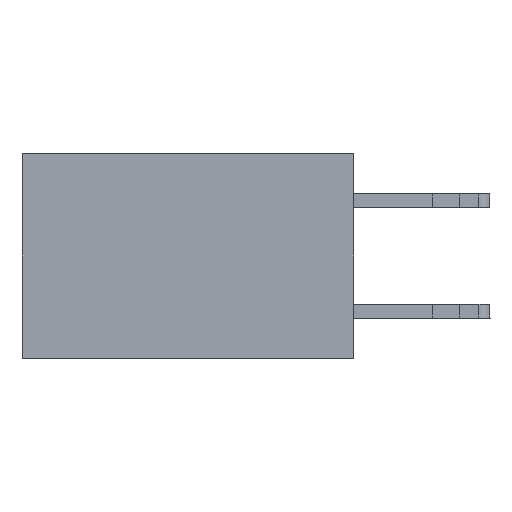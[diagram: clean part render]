
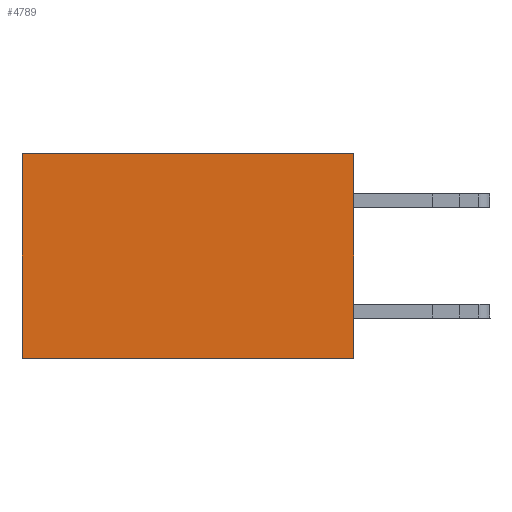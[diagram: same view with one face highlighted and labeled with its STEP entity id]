
A CAD part, left-side view. The second image highlights one B-rep face of the part: STEP entity #4789.
In plain terms, the highlighted planar face has unit normal (-1, 0, 0).
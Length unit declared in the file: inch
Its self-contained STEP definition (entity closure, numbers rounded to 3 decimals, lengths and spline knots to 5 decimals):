
#3145 = DIRECTION ( 'NONE',  ( 0., 1., 0. ) ) ;
#4263 = LINE ( 'NONE', #24356, #29850 ) ;
#4789 = ADVANCED_FACE ( 'NONE', ( #10942 ), #8909, .F. ) ;
#4837 = VERTEX_POINT ( 'NONE', #10345 ) ;
#5083 = LINE ( 'NONE', #15613, #27412 ) ;
#5341 = ORIENTED_EDGE ( 'NONE', *, *, #18465, .F. ) ;
#5527 = DIRECTION ( 'NONE',  ( 0., 0., -1. ) ) ;
#6210 = CARTESIAN_POINT ( 'NONE',  ( 0.2875, 0., 0. ) ) ;
#7867 = DIRECTION ( 'NONE',  ( 0., 0., -1. ) ) ;
#8586 = DIRECTION ( 'NONE',  ( 1., 0., 0. ) ) ;
#8909 = PLANE ( 'NONE',  #23403 ) ;
#9212 = EDGE_CURVE ( 'NONE', #30000, #29556, #5083, .T. ) ;
#9522 = EDGE_CURVE ( 'NONE', #29556, #21599, #14375, .T. ) ;
#10111 = CARTESIAN_POINT ( 'NONE',  ( 0.2875, 0.6, 0. ) ) ;
#10216 = EDGE_CURVE ( 'NONE', #30000, #4837, #15104, .T. ) ;
#10274 = VECTOR ( 'NONE', #5527, 39.37008 ) ;
#10345 = CARTESIAN_POINT ( 'NONE',  ( 0.2875, 0., -0.37 ) ) ;
#10942 = FACE_OUTER_BOUND ( 'NONE', #16728, .T. ) ;
#12621 = ORIENTED_EDGE ( 'NONE', *, *, #9212, .T. ) ;
#14375 = LINE ( 'NONE', #10111, #10274 ) ;
#15104 = LINE ( 'NONE', #17118, #18137 ) ;
#15613 = CARTESIAN_POINT ( 'NONE',  ( 0.2875, 0., 0. ) ) ;
#16728 = EDGE_LOOP ( 'NONE', ( #17444, #5341, #25704, #12621 ) ) ;
#17118 = CARTESIAN_POINT ( 'NONE',  ( 0.2875, 0., 0. ) ) ;
#17444 = ORIENTED_EDGE ( 'NONE', *, *, #9522, .T. ) ;
#18137 = VECTOR ( 'NONE', #7867, 39.37008 ) ;
#18465 = EDGE_CURVE ( 'NONE', #4837, #21599, #4263, .T. ) ;
#18467 = DIRECTION ( 'NONE',  ( 0., 0., -1. ) ) ;
#21599 = VERTEX_POINT ( 'NONE', #28707 ) ;
#23403 = AXIS2_PLACEMENT_3D ( 'NONE', #6210, #8586, #18467 ) ;
#24356 = CARTESIAN_POINT ( 'NONE',  ( 0.2875, 0., -0.37 ) ) ;
#25167 = DIRECTION ( 'NONE',  ( 0., 1., 0. ) ) ;
#25704 = ORIENTED_EDGE ( 'NONE', *, *, #10216, .F. ) ;
#27412 = VECTOR ( 'NONE', #25167, 39.37008 ) ;
#28413 = CARTESIAN_POINT ( 'NONE',  ( 0.2875, 0.6, 0. ) ) ;
#28707 = CARTESIAN_POINT ( 'NONE',  ( 0.2875, 0.6, -0.37 ) ) ;
#29556 = VERTEX_POINT ( 'NONE', #28413 ) ;
#29850 = VECTOR ( 'NONE', #3145, 39.37008 ) ;
#30000 = VERTEX_POINT ( 'NONE', #30121 ) ;
#30121 = CARTESIAN_POINT ( 'NONE',  ( 0.2875, 0., 0. ) ) ;
